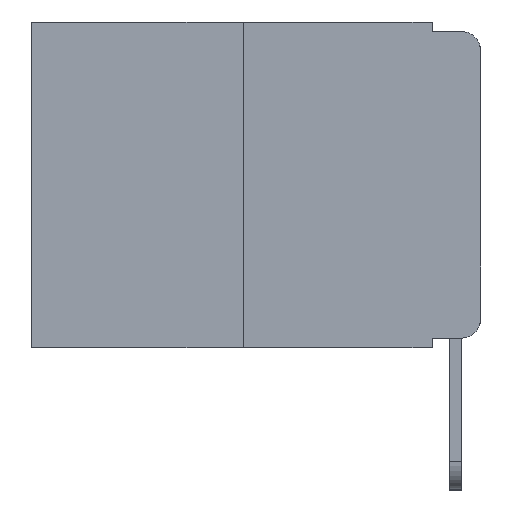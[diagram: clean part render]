
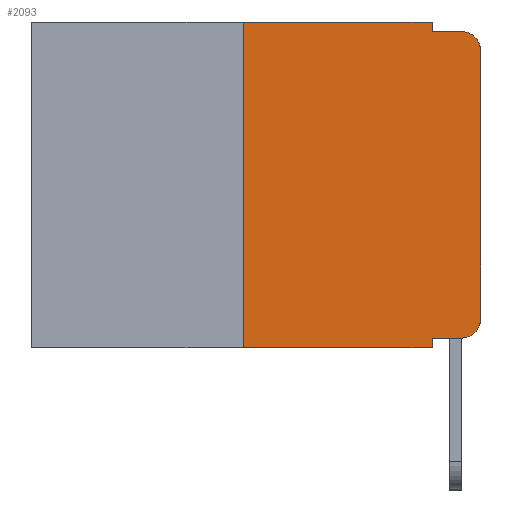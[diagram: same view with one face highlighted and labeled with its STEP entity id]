
A CAD part, left-side view. The second image highlights one B-rep face of the part: STEP entity #2093.
In plain terms, the highlighted planar face has unit normal (-1, 0, 0).
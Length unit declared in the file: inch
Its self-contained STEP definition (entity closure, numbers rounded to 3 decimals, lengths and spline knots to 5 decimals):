
#203 = DIRECTION ( 'NONE',  ( 0., -1., 0. ) ) ;
#738 = VECTOR ( 'NONE', #24462, 39.37008 ) ;
#1295 = CARTESIAN_POINT ( 'NONE',  ( 0., 0., -0.313 ) ) ;
#1498 = CARTESIAN_POINT ( 'NONE',  ( 0., 0.02, -0.313 ) ) ;
#1778 = EDGE_CURVE ( 'NONE', #9944, #19962, #22592, .T. ) ;
#2093 = ADVANCED_FACE ( 'NONE', ( #13341 ), #7005, .F. ) ;
#2199 = LINE ( 'NONE', #3175, #17795 ) ;
#2694 = CARTESIAN_POINT ( 'NONE',  ( 0., 0., -0.03 ) ) ;
#3168 = CARTESIAN_POINT ( 'NONE',  ( 0., 0.25, -0.343 ) ) ;
#3175 = CARTESIAN_POINT ( 'NONE',  ( 0., 0.473, -0.343 ) ) ;
#3693 = DIRECTION ( 'NONE',  ( 0., 0., -1. ) ) ;
#4034 = CARTESIAN_POINT ( 'NONE',  ( 0., 0.051, -0.333 ) ) ;
#4478 = ORIENTED_EDGE ( 'NONE', *, *, #22012, .F. ) ;
#4713 = DIRECTION ( 'NONE',  ( 0., -1., 0. ) ) ;
#4754 = CARTESIAN_POINT ( 'NONE',  ( 0., 0.051, 0. ) ) ;
#4760 = DIRECTION ( 'NONE',  ( 0., 0., -1. ) ) ;
#4803 = CIRCLE ( 'NONE', #15404, 0.02 ) ;
#5256 = DIRECTION ( 'NONE',  ( 0., -1., 0. ) ) ;
#6327 = EDGE_CURVE ( 'NONE', #23921, #16764, #20907, .T. ) ;
#6668 = CARTESIAN_POINT ( 'NONE',  ( 0., 0.25, 0. ) ) ;
#6923 = DIRECTION ( 'NONE',  ( 0., 0., -1. ) ) ;
#7005 = PLANE ( 'NONE',  #20389 ) ;
#7611 = CARTESIAN_POINT ( 'NONE',  ( 0., 0.051, 0. ) ) ;
#8107 = VECTOR ( 'NONE', #4760, 39.37008 ) ;
#8794 = ORIENTED_EDGE ( 'NONE', *, *, #12016, .T. ) ;
#9088 = ORIENTED_EDGE ( 'NONE', *, *, #15543, .T. ) ;
#9944 = VERTEX_POINT ( 'NONE', #7611 ) ;
#10322 = DIRECTION ( 'NONE',  ( -1., 0., 0. ) ) ;
#10612 = CARTESIAN_POINT ( 'NONE',  ( 0., 0.473, 0. ) ) ;
#10619 = ORIENTED_EDGE ( 'NONE', *, *, #12848, .T. ) ;
#10799 = VERTEX_POINT ( 'NONE', #25185 ) ;
#11575 = CARTESIAN_POINT ( 'NONE',  ( 0., 0.02, -0.01 ) ) ;
#11941 = DIRECTION ( 'NONE',  ( 0., 0., 1. ) ) ;
#12016 = EDGE_CURVE ( 'NONE', #18105, #16764, #2199, .T. ) ;
#12183 = VECTOR ( 'NONE', #20240, 39.37008 ) ;
#12199 = ORIENTED_EDGE ( 'NONE', *, *, #22751, .F. ) ;
#12777 = LINE ( 'NONE', #23975, #12183 ) ;
#12789 = ORIENTED_EDGE ( 'NONE', *, *, #20189, .F. ) ;
#12848 = EDGE_CURVE ( 'NONE', #18079, #13430, #4803, .T. ) ;
#13237 = CARTESIAN_POINT ( 'NONE',  ( 0., 0.051, 0. ) ) ;
#13341 = FACE_OUTER_BOUND ( 'NONE', #13460, .T. ) ;
#13430 = VERTEX_POINT ( 'NONE', #1295 ) ;
#13460 = EDGE_LOOP ( 'NONE', ( #17458, #9088, #4478, #16621, #12199, #12789, #8794, #14565, #20040, #10619 ) ) ;
#13784 = LINE ( 'NONE', #6668, #17545 ) ;
#14565 = ORIENTED_EDGE ( 'NONE', *, *, #6327, .F. ) ;
#15404 = AXIS2_PLACEMENT_3D ( 'NONE', #1498, #15423, #3693 ) ;
#15423 = DIRECTION ( 'NONE',  ( -1., 0., 0. ) ) ;
#15543 = EDGE_CURVE ( 'NONE', #20636, #20941, #22530, .T. ) ;
#16054 = VECTOR ( 'NONE', #203, 39.37008 ) ;
#16302 = LINE ( 'NONE', #10612, #20564 ) ;
#16621 = ORIENTED_EDGE ( 'NONE', *, *, #1778, .F. ) ;
#16764 = VERTEX_POINT ( 'NONE', #17063 ) ;
#16820 = CARTESIAN_POINT ( 'NONE',  ( 0., 0.02, -0.333 ) ) ;
#17063 = CARTESIAN_POINT ( 'NONE',  ( 0., 0.051, -0.343 ) ) ;
#17458 = ORIENTED_EDGE ( 'NONE', *, *, #21091, .T. ) ;
#17545 = VECTOR ( 'NONE', #21863, 39.37008 ) ;
#17795 = VECTOR ( 'NONE', #5256, 39.37008 ) ;
#17960 = CARTESIAN_POINT ( 'NONE',  ( 0., 0.051, -0.01 ) ) ;
#18079 = VERTEX_POINT ( 'NONE', #16820 ) ;
#18105 = VERTEX_POINT ( 'NONE', #3168 ) ;
#18369 = DIRECTION ( 'NONE',  ( 1., 0., 0. ) ) ;
#19201 = VECTOR ( 'NONE', #11941, 39.37008 ) ;
#19580 = EDGE_CURVE ( 'NONE', #23921, #18079, #12777, .T. ) ;
#19962 = VERTEX_POINT ( 'NONE', #21218 ) ;
#20040 = ORIENTED_EDGE ( 'NONE', *, *, #19580, .T. ) ;
#20189 = EDGE_CURVE ( 'NONE', #18105, #10799, #13784, .T. ) ;
#20240 = DIRECTION ( 'NONE',  ( 0., -1., 0. ) ) ;
#20389 = AXIS2_PLACEMENT_3D ( 'NONE', #21779, #18369, #6923 ) ;
#20481 = AXIS2_PLACEMENT_3D ( 'NONE', #21607, #10322, #23521 ) ;
#20564 = VECTOR ( 'NONE', #4713, 39.37008 ) ;
#20636 = VERTEX_POINT ( 'NONE', #2694 ) ;
#20894 = LINE ( 'NONE', #17960, #16054 ) ;
#20907 = LINE ( 'NONE', #13237, #738 ) ;
#20941 = VERTEX_POINT ( 'NONE', #11575 ) ;
#21091 = EDGE_CURVE ( 'NONE', #13430, #20636, #24774, .T. ) ;
#21214 = CARTESIAN_POINT ( 'NONE',  ( 0., 0., 0. ) ) ;
#21218 = CARTESIAN_POINT ( 'NONE',  ( 0., 0.051, -0.01 ) ) ;
#21607 = CARTESIAN_POINT ( 'NONE',  ( 0., 0.02, -0.03 ) ) ;
#21779 = CARTESIAN_POINT ( 'NONE',  ( 0., 0.473, 0. ) ) ;
#21863 = DIRECTION ( 'NONE',  ( 0., 0., 1. ) ) ;
#22012 = EDGE_CURVE ( 'NONE', #19962, #20941, #20894, .T. ) ;
#22530 = CIRCLE ( 'NONE', #20481, 0.02 ) ;
#22592 = LINE ( 'NONE', #4754, #8107 ) ;
#22751 = EDGE_CURVE ( 'NONE', #10799, #9944, #16302, .T. ) ;
#23521 = DIRECTION ( 'NONE',  ( 0., 0., -1. ) ) ;
#23921 = VERTEX_POINT ( 'NONE', #4034 ) ;
#23975 = CARTESIAN_POINT ( 'NONE',  ( 0., 0.051, -0.333 ) ) ;
#24462 = DIRECTION ( 'NONE',  ( 0., 0., -1. ) ) ;
#24774 = LINE ( 'NONE', #21214, #19201 ) ;
#25185 = CARTESIAN_POINT ( 'NONE',  ( 0., 0.25, 0. ) ) ;
